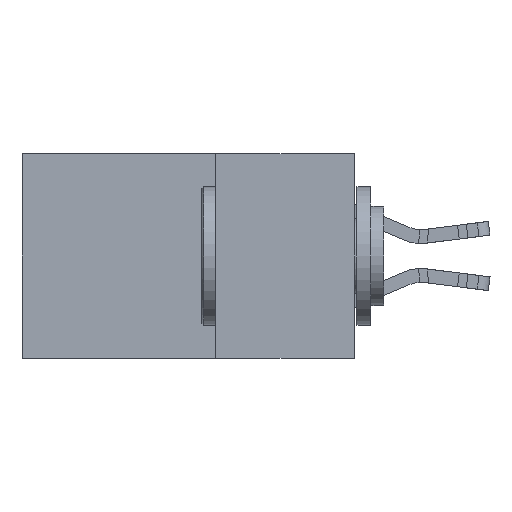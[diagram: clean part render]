
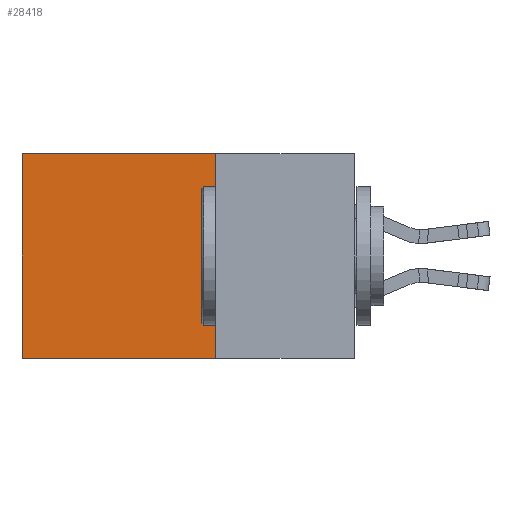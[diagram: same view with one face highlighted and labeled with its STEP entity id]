
A CAD part, left-side view. The second image highlights one B-rep face of the part: STEP entity #28418.
In plain terms, the highlighted planar face has unit normal (-1, 0, 0).
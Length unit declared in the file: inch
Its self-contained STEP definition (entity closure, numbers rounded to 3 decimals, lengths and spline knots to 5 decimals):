
#646 = PLANE ( 'NONE',  #24469 ) ;
#899 = ORIENTED_EDGE ( 'NONE', *, *, #10973, .F. ) ;
#2801 = ORIENTED_EDGE ( 'NONE', *, *, #21234, .T. ) ;
#3026 = DIRECTION ( 'NONE',  ( 0., 0., -1. ) ) ;
#3306 = LINE ( 'NONE', #17818, #19442 ) ;
#3746 = FACE_OUTER_BOUND ( 'NONE', #8524, .T. ) ;
#3938 = VERTEX_POINT ( 'NONE', #10674 ) ;
#6717 = CARTESIAN_POINT ( 'NONE',  ( 0.298, 0.6, 0. ) ) ;
#6961 = CARTESIAN_POINT ( 'NONE',  ( 0.298, 0.25, -0.37 ) ) ;
#8524 = EDGE_LOOP ( 'NONE', ( #2801, #10855, #899, #27915 ) ) ;
#8530 = LINE ( 'NONE', #6961, #29389 ) ;
#9445 = VERTEX_POINT ( 'NONE', #30201 ) ;
#9523 = EDGE_CURVE ( 'NONE', #29016, #9445, #8530, .T. ) ;
#10006 = CARTESIAN_POINT ( 'NONE',  ( 0.298, 0.25, 0. ) ) ;
#10674 = CARTESIAN_POINT ( 'NONE',  ( 0.298, 0.25, 0. ) ) ;
#10855 = ORIENTED_EDGE ( 'NONE', *, *, #9523, .F. ) ;
#10973 = EDGE_CURVE ( 'NONE', #3938, #29016, #3306, .T. ) ;
#11808 = DIRECTION ( 'NONE',  ( 0., 1., 0. ) ) ;
#12705 = EDGE_CURVE ( 'NONE', #3938, #30194, #25399, .T. ) ;
#13142 = CARTESIAN_POINT ( 'NONE',  ( 0.298, 0.25, 0. ) ) ;
#15735 = DIRECTION ( 'NONE',  ( 0., 1., 0. ) ) ;
#17818 = CARTESIAN_POINT ( 'NONE',  ( 0.298, 0.25, 0. ) ) ;
#19442 = VECTOR ( 'NONE', #24754, 39.37008 ) ;
#20228 = CARTESIAN_POINT ( 'NONE',  ( 0.298, 0.25, -0.37 ) ) ;
#20658 = VECTOR ( 'NONE', #15735, 39.37008 ) ;
#21234 = EDGE_CURVE ( 'NONE', #30194, #9445, #26703, .T. ) ;
#24469 = AXIS2_PLACEMENT_3D ( 'NONE', #10006, #26364, #3026 ) ;
#24754 = DIRECTION ( 'NONE',  ( 0., 0., -1. ) ) ;
#25399 = LINE ( 'NONE', #13142, #20658 ) ;
#26364 = DIRECTION ( 'NONE',  ( 1., 0., 0. ) ) ;
#26703 = LINE ( 'NONE', #6717, #29245 ) ;
#27718 = DIRECTION ( 'NONE',  ( 0., 0., -1. ) ) ;
#27915 = ORIENTED_EDGE ( 'NONE', *, *, #12705, .T. ) ;
#28151 = CARTESIAN_POINT ( 'NONE',  ( 0.298, 0.6, 0. ) ) ;
#28418 = ADVANCED_FACE ( 'NONE', ( #3746 ), #646, .F. ) ;
#29016 = VERTEX_POINT ( 'NONE', #20228 ) ;
#29245 = VECTOR ( 'NONE', #27718, 39.37008 ) ;
#29389 = VECTOR ( 'NONE', #11808, 39.37008 ) ;
#30194 = VERTEX_POINT ( 'NONE', #28151 ) ;
#30201 = CARTESIAN_POINT ( 'NONE',  ( 0.298, 0.6, -0.37 ) ) ;
